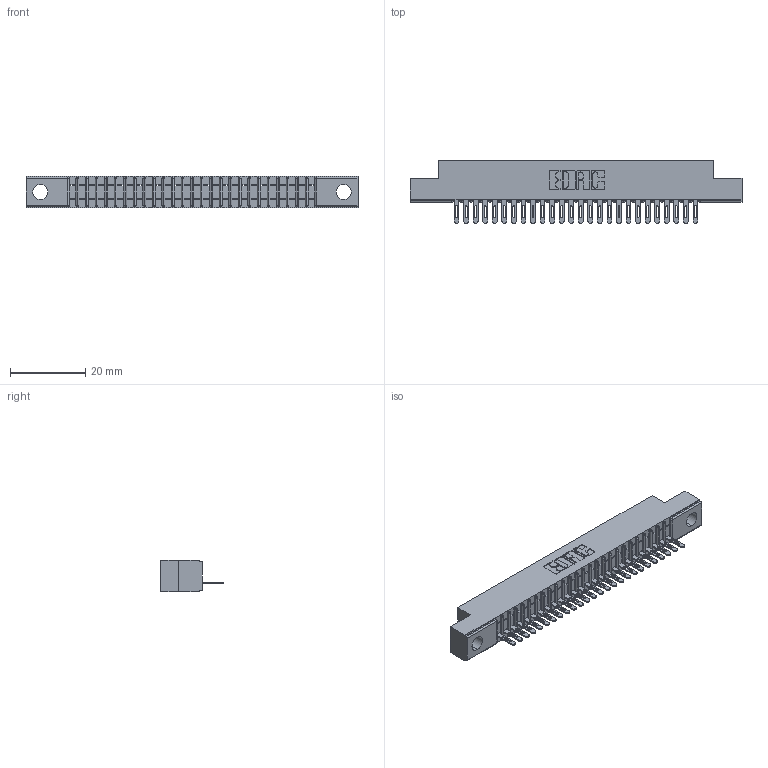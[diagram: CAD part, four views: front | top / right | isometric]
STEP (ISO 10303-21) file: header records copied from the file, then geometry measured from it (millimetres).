
FILE_DESCRIPTION (( 'STEP AP203' ), '1' );
FILE_NAME ('341-026-500-104.STEP', '2018-08-06T18:28:35', ( '' ), ( '' ), 'SwSTEP 2.0', 'SolidWorks 2016', '' );
FILE_SCHEMA (( 'CONFIG_CONTROL_DESIGN' ));
Length unit declared in the file: inch
Products named in the file (3): 341 Part_.156 (3.96) Dia Mounting Holes; 341-292-001_341-292-100; 341-026-500-104
Assembly tree (27 placements, depth 2):
  341-026-500-104
    341 Part_.156 (3.96) Dia Mounting Holes
    341-292-001_341-292-100  x26
Bounding box: 88.27 x 16.69 x 8.38 mm (x, y, z)
Volume: 4755.7 mm3; surface area: 9039.2 mm2
Topology: 27 solids, 27 shells, 2262 faces, 6514 edges, 4182 vertices
Faces by surface type: plane 1356, cylinder 802, sphere 54, torus 50
Entity records: 33191 total; most frequent: CARTESIAN_POINT 5634, ORIENTED_EDGE 5620, DIRECTION 5448, EDGE_CURVE 2810, LINE 2256, VECTOR 2256, VERTEX_POINT 1782, AXIS2_PLACEMENT_3D 1596
